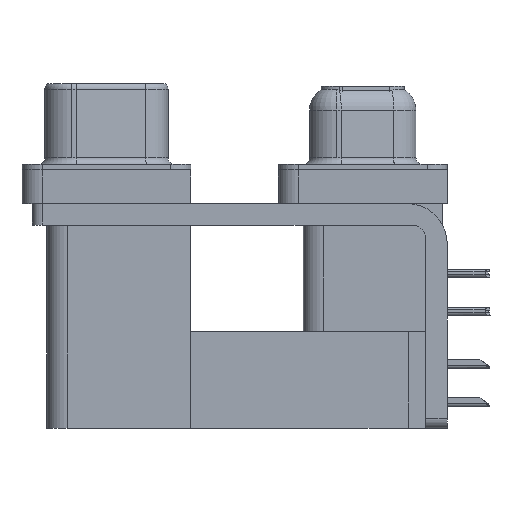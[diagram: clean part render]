
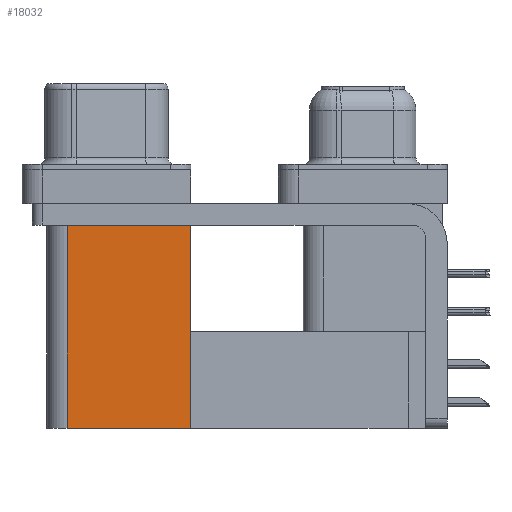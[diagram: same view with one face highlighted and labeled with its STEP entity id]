
A CAD part, left-side view. The second image highlights one B-rep face of the part: STEP entity #18032.
In plain terms, the highlighted planar face has unit normal (-1, 0, 0).
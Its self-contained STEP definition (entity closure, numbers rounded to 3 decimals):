
#397 = DIRECTION ( 'NONE',  ( 1., 0., 0. ) ) ;
#3347 = LINE ( 'NONE', #16865, #9275 ) ;
#9275 = VECTOR ( 'NONE', #30491, 1000. ) ;
#9518 = CARTESIAN_POINT ( 'NONE',  ( 3.765, 12.775, -2.5 ) ) ;
#9557 = ORIENTED_EDGE ( 'NONE', *, *, #34886, .T. ) ;
#11049 = EDGE_LOOP ( 'NONE', ( #9557, #41290, #32030, #25365 ) ) ;
#11918 = CARTESIAN_POINT ( 'NONE',  ( 3.765, 12.775, -19.2 ) ) ;
#13568 = VERTEX_POINT ( 'NONE', #22286 ) ;
#14121 = EDGE_CURVE ( 'NONE', #24766, #25078, #3347, .T. ) ;
#16865 = CARTESIAN_POINT ( 'NONE',  ( 3.765, 12.775, -19.2 ) ) ;
#17250 = DIRECTION ( 'NONE',  ( 0., 0., -1. ) ) ;
#17688 = FACE_OUTER_BOUND ( 'NONE', #11049, .T. ) ;
#18032 = ADVANCED_FACE ( 'NONE', ( #17688 ), #40857, .F. ) ;
#18931 = CARTESIAN_POINT ( 'NONE',  ( 3.765, 12.775, -19.2 ) ) ;
#22286 = CARTESIAN_POINT ( 'NONE',  ( 3.765, 12.775, -2.5 ) ) ;
#22374 = CARTESIAN_POINT ( 'NONE',  ( 3.765, 21.975, -2.5 ) ) ;
#22411 = LINE ( 'NONE', #9518, #32175 ) ;
#23132 = CARTESIAN_POINT ( 'NONE',  ( 3.765, 21.975, -19.2 ) ) ;
#24352 = EDGE_CURVE ( 'NONE', #24766, #13568, #25258, .T. ) ;
#24642 = DIRECTION ( 'NONE',  ( 0., 0., 1. ) ) ;
#24766 = VERTEX_POINT ( 'NONE', #18931 ) ;
#25078 = VERTEX_POINT ( 'NONE', #23132 ) ;
#25258 = LINE ( 'NONE', #11918, #38864 ) ;
#25365 = ORIENTED_EDGE ( 'NONE', *, *, #24352, .T. ) ;
#25983 = DIRECTION ( 'NONE',  ( 0., 1., 0. ) ) ;
#28221 = CARTESIAN_POINT ( 'NONE',  ( 3.765, 21.975, -19.2 ) ) ;
#30491 = DIRECTION ( 'NONE',  ( 0., 1., 0. ) ) ;
#31303 = CARTESIAN_POINT ( 'NONE',  ( 3.765, 12.775, -19.2 ) ) ;
#31436 = EDGE_CURVE ( 'NONE', #25078, #37451, #41789, .T. ) ;
#32030 = ORIENTED_EDGE ( 'NONE', *, *, #14121, .F. ) ;
#32175 = VECTOR ( 'NONE', #25983, 1000. ) ;
#34886 = EDGE_CURVE ( 'NONE', #13568, #37451, #22411, .T. ) ;
#35082 = DIRECTION ( 'NONE',  ( 0., 0., 1. ) ) ;
#37451 = VERTEX_POINT ( 'NONE', #22374 ) ;
#38864 = VECTOR ( 'NONE', #35082, 1000. ) ;
#40857 = PLANE ( 'NONE',  #43602 ) ;
#41290 = ORIENTED_EDGE ( 'NONE', *, *, #31436, .F. ) ;
#41315 = VECTOR ( 'NONE', #24642, 1000. ) ;
#41789 = LINE ( 'NONE', #28221, #41315 ) ;
#43602 = AXIS2_PLACEMENT_3D ( 'NONE', #31303, #397, #17250 ) ;
